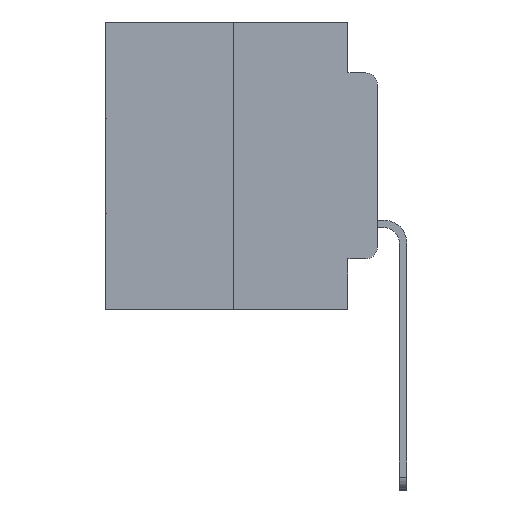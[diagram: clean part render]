
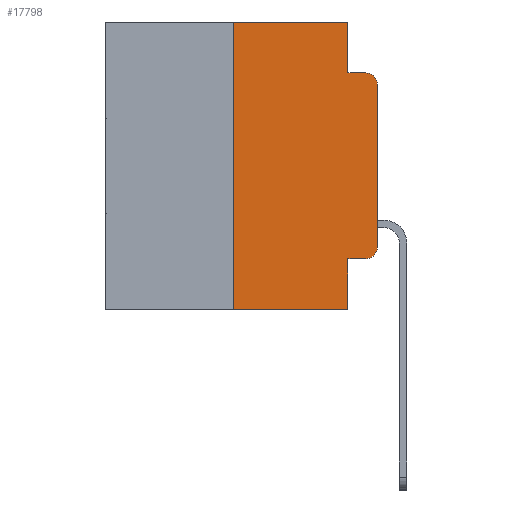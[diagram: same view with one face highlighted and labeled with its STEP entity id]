
A CAD part, left-side view. The second image highlights one B-rep face of the part: STEP entity #17798.
In plain terms, the highlighted planar face has unit normal (-1, 0, 0).
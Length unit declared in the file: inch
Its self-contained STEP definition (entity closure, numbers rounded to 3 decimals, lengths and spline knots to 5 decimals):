
#65 = EDGE_CURVE ( 'NONE', #27565, #6830, #27026, .T. ) ;
#92 = VERTEX_POINT ( 'NONE', #27308 ) ;
#488 = DIRECTION ( 'NONE',  ( 0., 0., -1. ) ) ;
#713 = DIRECTION ( 'NONE',  ( 0., 0., 1. ) ) ;
#747 = EDGE_CURVE ( 'NONE', #92, #2656, #12760, .T. ) ;
#750 = EDGE_CURVE ( 'NONE', #2656, #20574, #6516, .T. ) ;
#752 = EDGE_CURVE ( 'NONE', #27820, #20574, #18061, .T. ) ;
#754 = EDGE_CURVE ( 'NONE', #12978, #27820, #29675, .T. ) ;
#808 = EDGE_CURVE ( 'NONE', #27565, #16595, #27634, .T. ) ;
#858 = EDGE_CURVE ( 'NONE', #24815, #6830, #14508, .T. ) ;
#867 = EDGE_CURVE ( 'NONE', #24815, #23633, #8437, .T. ) ;
#911 = EDGE_CURVE ( 'NONE', #23633, #92, #23575, .T. ) ;
#1399 = DIRECTION ( 'NONE',  ( -1., 0., 0. ) ) ;
#1567 = ORIENTED_EDGE ( 'NONE', *, *, #752, .F. ) ;
#1630 = VECTOR ( 'NONE', #28709, 39.37008 ) ;
#2656 = VERTEX_POINT ( 'NONE', #4888 ) ;
#3101 = DIRECTION ( 'NONE',  ( 0., 0., -1. ) ) ;
#3203 = ORIENTED_EDGE ( 'NONE', *, *, #754, .F. ) ;
#3440 = FACE_OUTER_BOUND ( 'NONE', #9174, .T. ) ;
#4721 = LINE ( 'NONE', #10820, #11189 ) ;
#4888 = CARTESIAN_POINT ( 'NONE',  ( 0., 0., -0.1085 ) ) ;
#5581 = DIRECTION ( 'NONE',  ( 0., 0., 1. ) ) ;
#5693 = VECTOR ( 'NONE', #8127, 39.37008 ) ;
#6154 = DIRECTION ( 'NONE',  ( 0., 0., -1. ) ) ;
#6441 = ORIENTED_EDGE ( 'NONE', *, *, #867, .T. ) ;
#6516 = CIRCLE ( 'NONE', #27072, 0.02 ) ;
#6830 = VERTEX_POINT ( 'NONE', #9027 ) ;
#7088 = PLANE ( 'NONE',  #27623 ) ;
#7483 = CARTESIAN_POINT ( 'NONE',  ( 0., 0.25, -0.5 ) ) ;
#8005 = ORIENTED_EDGE ( 'NONE', *, *, #911, .T. ) ;
#8127 = DIRECTION ( 'NONE',  ( 0., -1., 0. ) ) ;
#8437 = LINE ( 'NONE', #20034, #1630 ) ;
#9027 = CARTESIAN_POINT ( 'NONE',  ( 0., 0.051, -0.5 ) ) ;
#9174 = EDGE_LOOP ( 'NONE', ( #29947, #13736, #1567, #3203, #27587, #28267, #23865, #29617, #6441, #8005 ) ) ;
#9269 = VECTOR ( 'NONE', #13635, 39.37008 ) ;
#9509 = DIRECTION ( 'NONE',  ( 0., 0., -1. ) ) ;
#10624 = VECTOR ( 'NONE', #713, 39.37008 ) ;
#10820 = CARTESIAN_POINT ( 'NONE',  ( 0., 0.473, 0. ) ) ;
#11189 = VECTOR ( 'NONE', #17631, 39.37008 ) ;
#11718 = CARTESIAN_POINT ( 'NONE',  ( 0., 0.473, 0. ) ) ;
#12760 = LINE ( 'NONE', #21686, #23923 ) ;
#12765 = CARTESIAN_POINT ( 'NONE',  ( 0., 0.051, 0. ) ) ;
#12978 = VERTEX_POINT ( 'NONE', #13909 ) ;
#13635 = DIRECTION ( 'NONE',  ( 0., -1., 0. ) ) ;
#13736 = ORIENTED_EDGE ( 'NONE', *, *, #750, .T. ) ;
#13909 = CARTESIAN_POINT ( 'NONE',  ( 0., 0.051, 0. ) ) ;
#14508 = LINE ( 'NONE', #24358, #26944 ) ;
#15021 = DIRECTION ( 'NONE',  ( -1., 0., 0. ) ) ;
#15791 = CARTESIAN_POINT ( 'NONE',  ( 0., 0.02, -0.3915 ) ) ;
#16595 = VERTEX_POINT ( 'NONE', #16773 ) ;
#16773 = CARTESIAN_POINT ( 'NONE',  ( 0., 0.25, 0. ) ) ;
#17631 = DIRECTION ( 'NONE',  ( 0., -1., 0. ) ) ;
#17798 = ADVANCED_FACE ( 'NONE', ( #3440 ), #7088, .F. ) ;
#18061 = LINE ( 'NONE', #19460, #5693 ) ;
#18092 = DIRECTION ( 'NONE',  ( 0., 0., -1. ) ) ;
#19460 = CARTESIAN_POINT ( 'NONE',  ( 0., 0.051, -0.0885 ) ) ;
#19540 = CARTESIAN_POINT ( 'NONE',  ( 0., 0.051, -0.0885 ) ) ;
#20034 = CARTESIAN_POINT ( 'NONE',  ( 0., 0.051, -0.4115 ) ) ;
#20263 = EDGE_CURVE ( 'NONE', #16595, #12978, #4721, .T. ) ;
#20574 = VERTEX_POINT ( 'NONE', #27396 ) ;
#21686 = CARTESIAN_POINT ( 'NONE',  ( 0., 0., 0. ) ) ;
#21974 = CARTESIAN_POINT ( 'NONE',  ( 0., 0.25, 0. ) ) ;
#22978 = DIRECTION ( 'NONE',  ( 1., 0., 0. ) ) ;
#23246 = VECTOR ( 'NONE', #3101, 39.37008 ) ;
#23575 = CIRCLE ( 'NONE', #23664, 0.02 ) ;
#23633 = VERTEX_POINT ( 'NONE', #26728 ) ;
#23664 = AXIS2_PLACEMENT_3D ( 'NONE', #15791, #1399, #18092 ) ;
#23865 = ORIENTED_EDGE ( 'NONE', *, *, #65, .T. ) ;
#23923 = VECTOR ( 'NONE', #5581, 39.37008 ) ;
#24358 = CARTESIAN_POINT ( 'NONE',  ( 0., 0.051, 0. ) ) ;
#24815 = VERTEX_POINT ( 'NONE', #27834 ) ;
#25880 = CARTESIAN_POINT ( 'NONE',  ( 0., 0.473, -0.5 ) ) ;
#26728 = CARTESIAN_POINT ( 'NONE',  ( 0., 0.02, -0.4115 ) ) ;
#26944 = VECTOR ( 'NONE', #6154, 39.37008 ) ;
#27026 = LINE ( 'NONE', #25880, #9269 ) ;
#27072 = AXIS2_PLACEMENT_3D ( 'NONE', #28228, #15021, #488 ) ;
#27308 = CARTESIAN_POINT ( 'NONE',  ( 0., 0., -0.3915 ) ) ;
#27396 = CARTESIAN_POINT ( 'NONE',  ( 0., 0.02, -0.0885 ) ) ;
#27565 = VERTEX_POINT ( 'NONE', #7483 ) ;
#27587 = ORIENTED_EDGE ( 'NONE', *, *, #20263, .F. ) ;
#27623 = AXIS2_PLACEMENT_3D ( 'NONE', #11718, #22978, #9509 ) ;
#27634 = LINE ( 'NONE', #21974, #10624 ) ;
#27820 = VERTEX_POINT ( 'NONE', #19540 ) ;
#27834 = CARTESIAN_POINT ( 'NONE',  ( 0., 0.051, -0.4115 ) ) ;
#28228 = CARTESIAN_POINT ( 'NONE',  ( 0., 0.02, -0.1085 ) ) ;
#28267 = ORIENTED_EDGE ( 'NONE', *, *, #808, .F. ) ;
#28709 = DIRECTION ( 'NONE',  ( 0., -1., 0. ) ) ;
#29617 = ORIENTED_EDGE ( 'NONE', *, *, #858, .F. ) ;
#29675 = LINE ( 'NONE', #12765, #23246 ) ;
#29947 = ORIENTED_EDGE ( 'NONE', *, *, #747, .T. ) ;
